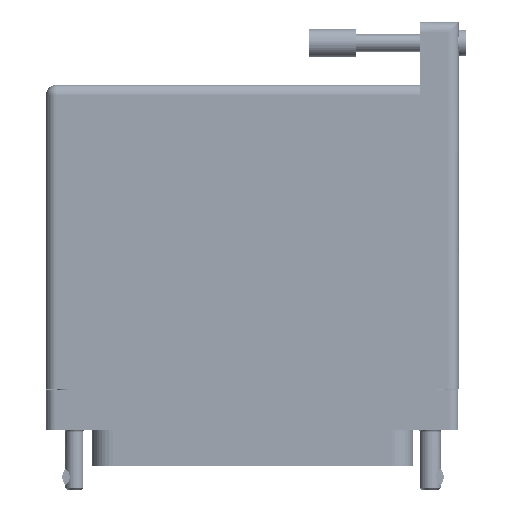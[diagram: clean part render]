
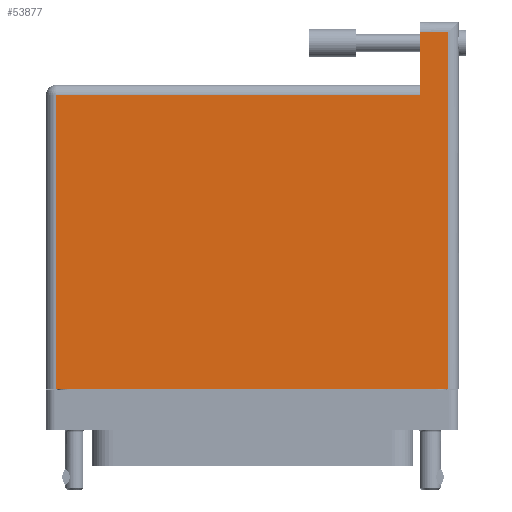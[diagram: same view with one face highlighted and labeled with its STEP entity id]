
A CAD part, front view. The second image highlights one B-rep face of the part: STEP entity #53877.
In plain terms, the highlighted face is planar.
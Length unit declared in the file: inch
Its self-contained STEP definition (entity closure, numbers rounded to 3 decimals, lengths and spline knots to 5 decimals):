
#2401 = EDGE_CURVE ( 'NONE', #5678, #30418, #47638, .T. ) ;
#3675 = FACE_OUTER_BOUND ( 'NONE', #51669, .T. ) ;
#4908 = CARTESIAN_POINT ( 'NONE',  ( 1.1215, 2.35, 0.765 ) ) ;
#5280 = LINE ( 'NONE', #11415, #84727 ) ;
#5678 = VERTEX_POINT ( 'NONE', #48533 ) ;
#7116 = VERTEX_POINT ( 'NONE', #53088 ) ;
#8593 = EDGE_CURVE ( 'NONE', #42350, #7116, #28656, .T. ) ;
#9247 = CARTESIAN_POINT ( 'NONE',  ( 1.1215, 1.86, 0.765 ) ) ;
#11415 = CARTESIAN_POINT ( 'NONE',  ( -1.3775, -0.1, 0.765 ) ) ;
#17629 = CARTESIAN_POINT ( 'NONE',  ( -1.3075, -0.1, 0.765 ) ) ;
#18934 = EDGE_CURVE ( 'NONE', #61552, #5678, #36237, .T. ) ;
#19480 = CARTESIAN_POINT ( 'NONE',  ( -1.3775, 2.28, 0.765 ) ) ;
#25457 = CARTESIAN_POINT ( 'NONE',  ( -1.3775, 1.93, 0.765 ) ) ;
#26615 = CARTESIAN_POINT ( 'NONE',  ( 1.3075, 2.35, 0.765 ) ) ;
#26959 = DIRECTION ( 'NONE',  ( 0., 1., 0. ) ) ;
#27722 = ORIENTED_EDGE ( 'NONE', *, *, #35928, .T. ) ;
#28656 = LINE ( 'NONE', #19480, #31159 ) ;
#30418 = VERTEX_POINT ( 'NONE', #17629 ) ;
#31159 = VECTOR ( 'NONE', #91333, 39.37008 ) ;
#32100 = PLANE ( 'NONE',  #65398 ) ;
#32420 = CARTESIAN_POINT ( 'NONE',  ( 1.3075, -0.1, 0.765 ) ) ;
#35928 = EDGE_CURVE ( 'NONE', #30418, #50877, #5280, .T. ) ;
#36237 = LINE ( 'NONE', #50696, #66040 ) ;
#42350 = VERTEX_POINT ( 'NONE', #99244 ) ;
#42701 = CARTESIAN_POINT ( 'NONE',  ( -1.3075, -0.1, 0.765 ) ) ;
#47638 = LINE ( 'NONE', #42701, #87405 ) ;
#48533 = CARTESIAN_POINT ( 'NONE',  ( -1.3075, 1.86, 0.765 ) ) ;
#50255 = LINE ( 'NONE', #26615, #81356 ) ;
#50696 = CARTESIAN_POINT ( 'NONE',  ( -1.3775, 1.86, 0.765 ) ) ;
#50877 = VERTEX_POINT ( 'NONE', #32420 ) ;
#51031 = DIRECTION ( 'NONE',  ( -1., 0., 0. ) ) ;
#51286 = DIRECTION ( 'NONE',  ( 1., 0., 0. ) ) ;
#51359 = ORIENTED_EDGE ( 'NONE', *, *, #2401, .T. ) ;
#51669 = EDGE_LOOP ( 'NONE', ( #52259, #78018, #51359, #27722, #91418, #99172 ) ) ;
#52259 = ORIENTED_EDGE ( 'NONE', *, *, #82839, .T. ) ;
#53088 = CARTESIAN_POINT ( 'NONE',  ( 1.1215, 2.28, 0.765 ) ) ;
#53877 = ADVANCED_FACE ( 'NONE', ( #3675 ), #32100, .F. ) ;
#55722 = DIRECTION ( 'NONE',  ( 0., 0., -1. ) ) ;
#61489 = VECTOR ( 'NONE', #84349, 39.37008 ) ;
#61552 = VERTEX_POINT ( 'NONE', #9247 ) ;
#65398 = AXIS2_PLACEMENT_3D ( 'NONE', #25457, #55722, #80039 ) ;
#65424 = EDGE_CURVE ( 'NONE', #50877, #42350, #50255, .T. ) ;
#66040 = VECTOR ( 'NONE', #51031, 39.37008 ) ;
#73596 = DIRECTION ( 'NONE',  ( 0., -1., 0. ) ) ;
#78018 = ORIENTED_EDGE ( 'NONE', *, *, #18934, .T. ) ;
#80039 = DIRECTION ( 'NONE',  ( -1., 0., 0. ) ) ;
#80967 = LINE ( 'NONE', #4908, #61489 ) ;
#81356 = VECTOR ( 'NONE', #26959, 39.37008 ) ;
#82839 = EDGE_CURVE ( 'NONE', #7116, #61552, #80967, .T. ) ;
#84349 = DIRECTION ( 'NONE',  ( 0., -1., 0. ) ) ;
#84727 = VECTOR ( 'NONE', #51286, 39.37008 ) ;
#87405 = VECTOR ( 'NONE', #73596, 39.37008 ) ;
#91333 = DIRECTION ( 'NONE',  ( -1., 0., 0. ) ) ;
#91418 = ORIENTED_EDGE ( 'NONE', *, *, #65424, .T. ) ;
#99172 = ORIENTED_EDGE ( 'NONE', *, *, #8593, .T. ) ;
#99244 = CARTESIAN_POINT ( 'NONE',  ( 1.3075, 2.28, 0.765 ) ) ;
